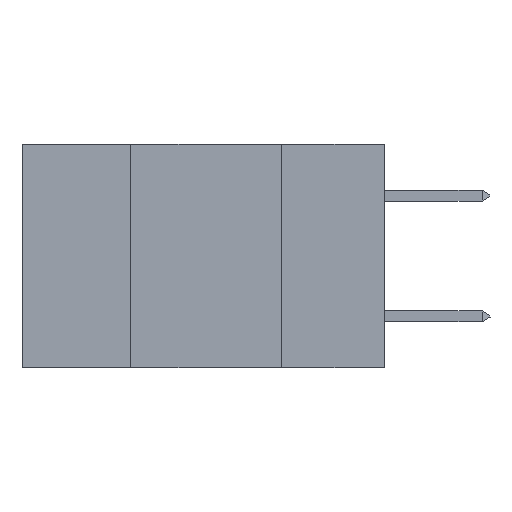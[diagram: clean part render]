
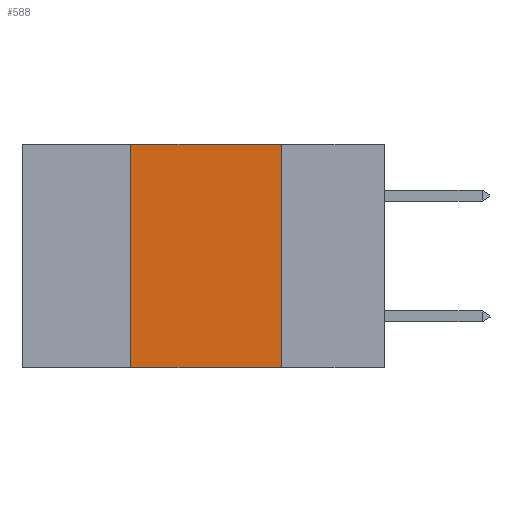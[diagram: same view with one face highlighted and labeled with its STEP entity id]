
A CAD part, left-side view. The second image highlights one B-rep face of the part: STEP entity #588.
In plain terms, the highlighted planar face has unit normal (-1, 0, 0).
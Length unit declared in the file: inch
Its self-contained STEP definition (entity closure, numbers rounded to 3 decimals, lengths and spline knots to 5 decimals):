
#578 = EDGE_LOOP ( 'NONE', ( #12705, #13116, #6629, #8243 ) ) ;
#588 = ADVANCED_FACE ( 'NONE', ( #12087 ), #3879, .F. ) ;
#631 = VERTEX_POINT ( 'NONE', #14084 ) ;
#2062 = EDGE_CURVE ( 'NONE', #631, #6331, #8424, .T. ) ;
#2629 = LINE ( 'NONE', #8893, #5057 ) ;
#3346 = CARTESIAN_POINT ( 'NONE',  ( 0., 0.17, 0. ) ) ;
#3879 = PLANE ( 'NONE',  #7374 ) ;
#4042 = VERTEX_POINT ( 'NONE', #3346 ) ;
#4954 = CARTESIAN_POINT ( 'NONE',  ( 0., 0.6, -0.37 ) ) ;
#5057 = VECTOR ( 'NONE', #11999, 39.37008 ) ;
#6140 = DIRECTION ( 'NONE',  ( 1., 0., 0. ) ) ;
#6331 = VERTEX_POINT ( 'NONE', #8420 ) ;
#6379 = VECTOR ( 'NONE', #12521, 39.37008 ) ;
#6569 = LINE ( 'NONE', #9677, #10529 ) ;
#6629 = ORIENTED_EDGE ( 'NONE', *, *, #13842, .F. ) ;
#7374 = AXIS2_PLACEMENT_3D ( 'NONE', #11613, #6140, #13866 ) ;
#7681 = DIRECTION ( 'NONE',  ( 0., -1., 0. ) ) ;
#7848 = EDGE_CURVE ( 'NONE', #4042, #6331, #10385, .T. ) ;
#8243 = ORIENTED_EDGE ( 'NONE', *, *, #2062, .T. ) ;
#8261 = CARTESIAN_POINT ( 'NONE',  ( 0., 0.17, 0. ) ) ;
#8348 = DIRECTION ( 'NONE',  ( 0., 0., -1. ) ) ;
#8420 = CARTESIAN_POINT ( 'NONE',  ( 0., 0.17, -0.37 ) ) ;
#8424 = LINE ( 'NONE', #4954, #6379 ) ;
#8853 = EDGE_CURVE ( 'NONE', #12916, #4042, #6569, .T. ) ;
#8893 = CARTESIAN_POINT ( 'NONE',  ( 0., 0.42, 0. ) ) ;
#9677 = CARTESIAN_POINT ( 'NONE',  ( 0., 0.6, 0. ) ) ;
#10385 = LINE ( 'NONE', #8261, #10721 ) ;
#10529 = VECTOR ( 'NONE', #7681, 39.37008 ) ;
#10721 = VECTOR ( 'NONE', #8348, 39.37008 ) ;
#11055 = CARTESIAN_POINT ( 'NONE',  ( 0., 0.42, 0. ) ) ;
#11613 = CARTESIAN_POINT ( 'NONE',  ( 0., 0.6, 0. ) ) ;
#11999 = DIRECTION ( 'NONE',  ( 0., 0., 1. ) ) ;
#12087 = FACE_OUTER_BOUND ( 'NONE', #578, .T. ) ;
#12521 = DIRECTION ( 'NONE',  ( 0., -1., 0. ) ) ;
#12705 = ORIENTED_EDGE ( 'NONE', *, *, #7848, .F. ) ;
#12916 = VERTEX_POINT ( 'NONE', #11055 ) ;
#13116 = ORIENTED_EDGE ( 'NONE', *, *, #8853, .F. ) ;
#13842 = EDGE_CURVE ( 'NONE', #631, #12916, #2629, .T. ) ;
#13866 = DIRECTION ( 'NONE',  ( 0., 0., -1. ) ) ;
#14084 = CARTESIAN_POINT ( 'NONE',  ( 0., 0.42, -0.37 ) ) ;
